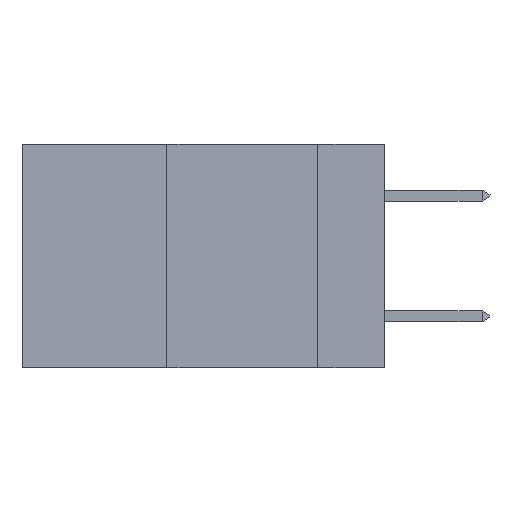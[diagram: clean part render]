
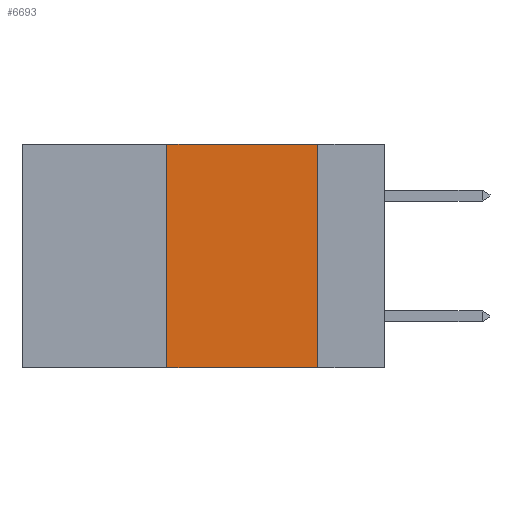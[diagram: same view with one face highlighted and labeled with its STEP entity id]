
A CAD part, left-side view. The second image highlights one B-rep face of the part: STEP entity #6693.
In plain terms, the highlighted planar face has unit normal (-1, 0, 0).
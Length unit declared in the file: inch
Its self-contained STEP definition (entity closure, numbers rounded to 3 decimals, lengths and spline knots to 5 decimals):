
#114 = CARTESIAN_POINT ( 'NONE',  ( 0., 0.11, 0. ) ) ;
#188 = DIRECTION ( 'NONE',  ( 0., 0., -1. ) ) ;
#224 = LINE ( 'NONE', #18728, #4685 ) ;
#670 = VECTOR ( 'NONE', #3828, 39.37008 ) ;
#1237 = EDGE_CURVE ( 'NONE', #18067, #16236, #224, .T. ) ;
#1391 = LINE ( 'NONE', #17003, #12397 ) ;
#3601 = DIRECTION ( 'NONE',  ( 0., 0., -1. ) ) ;
#3828 = DIRECTION ( 'NONE',  ( 0., -1., 0. ) ) ;
#4081 = CARTESIAN_POINT ( 'NONE',  ( 0., 0.11, -0.37 ) ) ;
#4144 = ORIENTED_EDGE ( 'NONE', *, *, #5801, .F. ) ;
#4685 = VECTOR ( 'NONE', #15720, 39.37008 ) ;
#5801 = EDGE_CURVE ( 'NONE', #17385, #16236, #13034, .T. ) ;
#6382 = EDGE_LOOP ( 'NONE', ( #4144, #13184, #19840, #6833 ) ) ;
#6693 = ADVANCED_FACE ( 'NONE', ( #18750 ), #11050, .F. ) ;
#6833 = ORIENTED_EDGE ( 'NONE', *, *, #1237, .T. ) ;
#6971 = DIRECTION ( 'NONE',  ( 1., 0., 0. ) ) ;
#7085 = LINE ( 'NONE', #13982, #670 ) ;
#8213 = EDGE_CURVE ( 'NONE', #18067, #8854, #1391, .T. ) ;
#8853 = CARTESIAN_POINT ( 'NONE',  ( 0., 0.11, 0. ) ) ;
#8854 = VERTEX_POINT ( 'NONE', #8996 ) ;
#8996 = CARTESIAN_POINT ( 'NONE',  ( 0., 0.36, 0. ) ) ;
#9531 = AXIS2_PLACEMENT_3D ( 'NONE', #12614, #6971, #3601 ) ;
#10574 = VECTOR ( 'NONE', #188, 39.37008 ) ;
#11050 = PLANE ( 'NONE',  #9531 ) ;
#12397 = VECTOR ( 'NONE', #14033, 39.37008 ) ;
#12614 = CARTESIAN_POINT ( 'NONE',  ( 0., 0.6, 0. ) ) ;
#13034 = LINE ( 'NONE', #114, #10574 ) ;
#13162 = CARTESIAN_POINT ( 'NONE',  ( 0., 0.36, -0.37 ) ) ;
#13184 = ORIENTED_EDGE ( 'NONE', *, *, #14423, .F. ) ;
#13982 = CARTESIAN_POINT ( 'NONE',  ( 0., 0.6, 0. ) ) ;
#14033 = DIRECTION ( 'NONE',  ( 0., 0., 1. ) ) ;
#14423 = EDGE_CURVE ( 'NONE', #8854, #17385, #7085, .T. ) ;
#15720 = DIRECTION ( 'NONE',  ( 0., -1., 0. ) ) ;
#16236 = VERTEX_POINT ( 'NONE', #4081 ) ;
#17003 = CARTESIAN_POINT ( 'NONE',  ( 0., 0.36, 0. ) ) ;
#17385 = VERTEX_POINT ( 'NONE', #8853 ) ;
#18067 = VERTEX_POINT ( 'NONE', #13162 ) ;
#18728 = CARTESIAN_POINT ( 'NONE',  ( 0., 0.6, -0.37 ) ) ;
#18750 = FACE_OUTER_BOUND ( 'NONE', #6382, .T. ) ;
#19840 = ORIENTED_EDGE ( 'NONE', *, *, #8213, .F. ) ;
